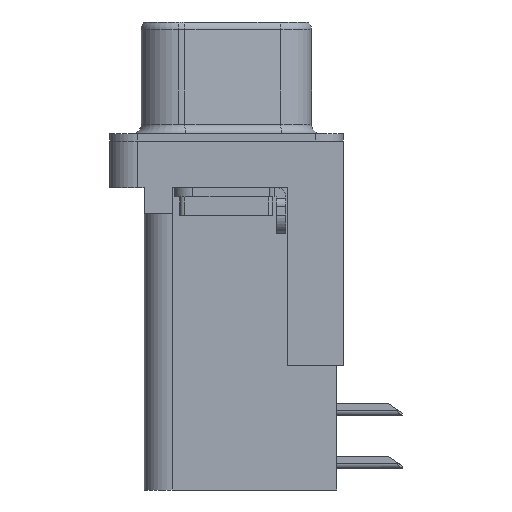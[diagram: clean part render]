
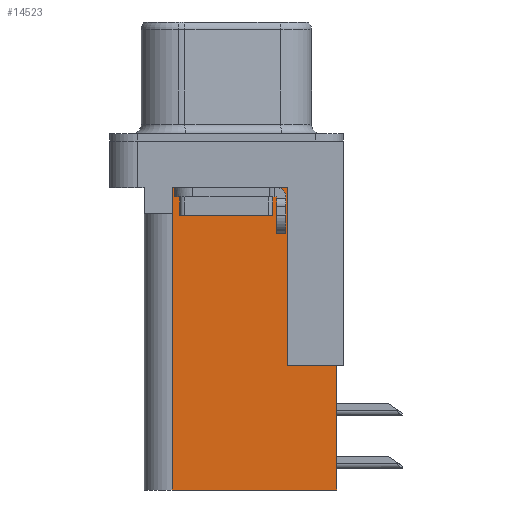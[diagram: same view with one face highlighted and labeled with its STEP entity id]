
A CAD part, left-side view. The second image highlights one B-rep face of the part: STEP entity #14523.
In plain terms, the highlighted planar face has unit normal (-1, 0, 0).
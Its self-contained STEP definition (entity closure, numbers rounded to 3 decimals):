
#337 = LINE ( 'NONE', #6323, #18150 ) ;
#529 = ORIENTED_EDGE ( 'NONE', *, *, #2991, .F. ) ;
#568 = EDGE_CURVE ( 'NONE', #4520, #12390, #6082, .T. ) ;
#582 = ORIENTED_EDGE ( 'NONE', *, *, #16918, .F. ) ;
#686 = VERTEX_POINT ( 'NONE', #6173 ) ;
#1016 = VECTOR ( 'NONE', #14698, 1000. ) ;
#1075 = EDGE_CURVE ( 'NONE', #11587, #10020, #18066, .T. ) ;
#1701 = EDGE_CURVE ( 'NONE', #14572, #9295, #17301, .T. ) ;
#1964 = ORIENTED_EDGE ( 'NONE', *, *, #1701, .T. ) ;
#2444 = VECTOR ( 'NONE', #4035, 1000. ) ;
#2991 = EDGE_CURVE ( 'NONE', #686, #4520, #337, .T. ) ;
#3628 = ORIENTED_EDGE ( 'NONE', *, *, #568, .F. ) ;
#4035 = DIRECTION ( 'NONE',  ( 0., 0., -1. ) ) ;
#4520 = VERTEX_POINT ( 'NONE', #6376 ) ;
#4541 = CARTESIAN_POINT ( 'NONE',  ( 3.765, 0., -3.9 ) ) ;
#4565 = CARTESIAN_POINT ( 'NONE',  ( 3.765, -3.295, -2.5 ) ) ;
#4663 = CARTESIAN_POINT ( 'NONE',  ( 3.765, 2.895, -3.9 ) ) ;
#5578 = CARTESIAN_POINT ( 'NONE',  ( 3.765, -3.295, -18.76 ) ) ;
#5777 = CARTESIAN_POINT ( 'NONE',  ( 3.765, -3.295, -18.76 ) ) ;
#6082 = LINE ( 'NONE', #17205, #9503 ) ;
#6140 = EDGE_CURVE ( 'NONE', #10020, #12694, #18393, .T. ) ;
#6173 = CARTESIAN_POINT ( 'NONE',  ( 3.765, -5.925, -18.76 ) ) ;
#6323 = CARTESIAN_POINT ( 'NONE',  ( 3.765, -3.295, -18.76 ) ) ;
#6376 = CARTESIAN_POINT ( 'NONE',  ( 3.765, 2.925, -18.76 ) ) ;
#6528 = VECTOR ( 'NONE', #10100, 1000. ) ;
#6751 = ORIENTED_EDGE ( 'NONE', *, *, #6140, .T. ) ;
#6929 = EDGE_CURVE ( 'NONE', #9295, #12390, #14080, .T. ) ;
#7057 = DIRECTION ( 'NONE',  ( 0., 1., 0. ) ) ;
#7475 = DIRECTION ( 'NONE',  ( 0., 1., 0. ) ) ;
#7638 = CARTESIAN_POINT ( 'NONE',  ( 3.765, 2.895, -3.9 ) ) ;
#7773 = CARTESIAN_POINT ( 'NONE',  ( 3.765, -6.295, -12.05 ) ) ;
#8189 = DIRECTION ( 'NONE',  ( 0., 1., 0. ) ) ;
#8206 = LINE ( 'NONE', #4565, #1016 ) ;
#8333 = EDGE_LOOP ( 'NONE', ( #10614, #1964, #8850, #3628, #529, #582, #18209, #6751 ) ) ;
#8454 = PLANE ( 'NONE',  #17059 ) ;
#8850 = ORIENTED_EDGE ( 'NONE', *, *, #6929, .T. ) ;
#9295 = VERTEX_POINT ( 'NONE', #4663 ) ;
#9503 = VECTOR ( 'NONE', #12073, 1000. ) ;
#9557 = CARTESIAN_POINT ( 'NONE',  ( 3.765, -5.925, -12.05 ) ) ;
#9821 = VECTOR ( 'NONE', #7475, 1000. ) ;
#10020 = VERTEX_POINT ( 'NONE', #14715 ) ;
#10100 = DIRECTION ( 'NONE',  ( 0., 1., 0. ) ) ;
#10614 = ORIENTED_EDGE ( 'NONE', *, *, #14709, .T. ) ;
#10953 = FACE_OUTER_BOUND ( 'NONE', #8333, .T. ) ;
#11184 = CARTESIAN_POINT ( 'NONE',  ( 3.765, -3.295, -2.5 ) ) ;
#11311 = CARTESIAN_POINT ( 'NONE',  ( 3.765, -5.925, -2. ) ) ;
#11587 = VERTEX_POINT ( 'NONE', #9557 ) ;
#12073 = DIRECTION ( 'NONE',  ( 0., 0., 1. ) ) ;
#12390 = VERTEX_POINT ( 'NONE', #14895 ) ;
#12694 = VERTEX_POINT ( 'NONE', #11184 ) ;
#13185 = VECTOR ( 'NONE', #15930, 1000. ) ;
#13881 = VECTOR ( 'NONE', #15755, 1000. ) ;
#14080 = LINE ( 'NONE', #4541, #9821 ) ;
#14330 = CARTESIAN_POINT ( 'NONE',  ( 3.765, 2.895, -2.5 ) ) ;
#14523 = ADVANCED_FACE ( 'NONE', ( #10953 ), #8454, .F. ) ;
#14572 = VERTEX_POINT ( 'NONE', #14330 ) ;
#14698 = DIRECTION ( 'NONE',  ( 0., 1., 0. ) ) ;
#14709 = EDGE_CURVE ( 'NONE', #12694, #14572, #8206, .T. ) ;
#14715 = CARTESIAN_POINT ( 'NONE',  ( 3.765, -3.295, -12.05 ) ) ;
#14895 = CARTESIAN_POINT ( 'NONE',  ( 3.765, 2.925, -3.9 ) ) ;
#15742 = DIRECTION ( 'NONE',  ( 1., 0., 0. ) ) ;
#15755 = DIRECTION ( 'NONE',  ( 0., 0., -1. ) ) ;
#15930 = DIRECTION ( 'NONE',  ( 0., 0., 1. ) ) ;
#16918 = EDGE_CURVE ( 'NONE', #11587, #686, #17380, .T. ) ;
#17059 = AXIS2_PLACEMENT_3D ( 'NONE', #5578, #15742, #7057 ) ;
#17205 = CARTESIAN_POINT ( 'NONE',  ( 3.765, 2.925, -18.76 ) ) ;
#17301 = LINE ( 'NONE', #7638, #13881 ) ;
#17380 = LINE ( 'NONE', #11311, #2444 ) ;
#18066 = LINE ( 'NONE', #7773, #6528 ) ;
#18150 = VECTOR ( 'NONE', #8189, 1000. ) ;
#18209 = ORIENTED_EDGE ( 'NONE', *, *, #1075, .T. ) ;
#18393 = LINE ( 'NONE', #5777, #13185 ) ;
